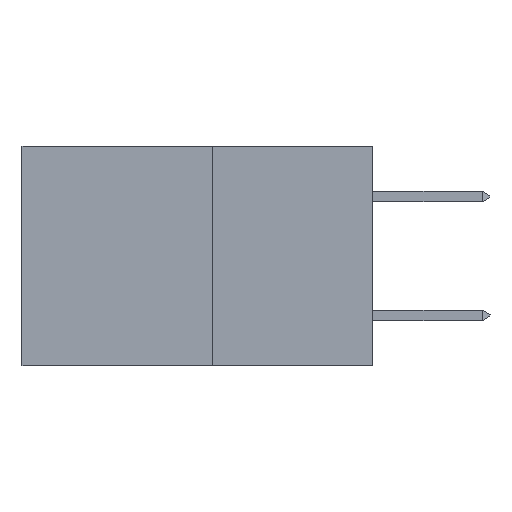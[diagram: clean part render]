
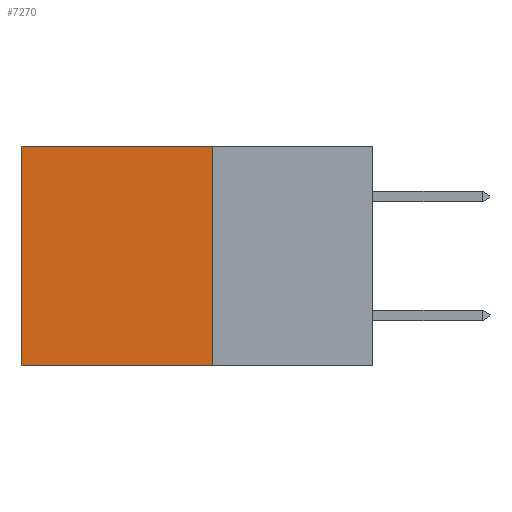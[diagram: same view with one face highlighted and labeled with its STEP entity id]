
A CAD part, left-side view. The second image highlights one B-rep face of the part: STEP entity #7270.
In plain terms, the highlighted planar face has unit normal (-1, 0, 0).
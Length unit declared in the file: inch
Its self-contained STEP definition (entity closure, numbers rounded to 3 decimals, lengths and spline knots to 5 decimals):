
#323 = CARTESIAN_POINT ( 'NONE',  ( 0.277, 0.59, 0. ) ) ;
#431 = EDGE_LOOP ( 'NONE', ( #13300, #8827, #19521, #10023 ) ) ;
#618 = EDGE_CURVE ( 'NONE', #21297, #9839, #15740, .T. ) ;
#1033 = DIRECTION ( 'NONE',  ( 0., 0., -1. ) ) ;
#2164 = CARTESIAN_POINT ( 'NONE',  ( 0.277, 0.59, -0.37 ) ) ;
#3839 = FACE_OUTER_BOUND ( 'NONE', #431, .T. ) ;
#4172 = VERTEX_POINT ( 'NONE', #14036 ) ;
#4552 = VECTOR ( 'NONE', #4832, 39.37008 ) ;
#4832 = DIRECTION ( 'NONE',  ( 0., 0., -1. ) ) ;
#5787 = VERTEX_POINT ( 'NONE', #10818 ) ;
#7270 = ADVANCED_FACE ( 'NONE', ( #3839 ), #23300, .F. ) ;
#8087 = DIRECTION ( 'NONE',  ( 0., 0., -1. ) ) ;
#8827 = ORIENTED_EDGE ( 'NONE', *, *, #24014, .F. ) ;
#9708 = LINE ( 'NONE', #20129, #4552 ) ;
#9839 = VERTEX_POINT ( 'NONE', #2164 ) ;
#10023 = ORIENTED_EDGE ( 'NONE', *, *, #21943, .T. ) ;
#10700 = VECTOR ( 'NONE', #8087, 39.37008 ) ;
#10818 = CARTESIAN_POINT ( 'NONE',  ( 0.277, 0.27, -0.37 ) ) ;
#13300 = ORIENTED_EDGE ( 'NONE', *, *, #618, .T. ) ;
#13712 = CARTESIAN_POINT ( 'NONE',  ( 0.277, 0.27, 0. ) ) ;
#14000 = LINE ( 'NONE', #23015, #24183 ) ;
#14036 = CARTESIAN_POINT ( 'NONE',  ( 0.277, 0.27, 0. ) ) ;
#15620 = DIRECTION ( 'NONE',  ( 0., 1., 0. ) ) ;
#15740 = LINE ( 'NONE', #17177, #10700 ) ;
#15846 = VECTOR ( 'NONE', #15620, 39.37008 ) ;
#17177 = CARTESIAN_POINT ( 'NONE',  ( 0.277, 0.59, -0.37 ) ) ;
#17493 = EDGE_CURVE ( 'NONE', #4172, #5787, #9708, .T. ) ;
#18399 = AXIS2_PLACEMENT_3D ( 'NONE', #19696, #23014, #1033 ) ;
#19521 = ORIENTED_EDGE ( 'NONE', *, *, #17493, .F. ) ;
#19696 = CARTESIAN_POINT ( 'NONE',  ( 0.277, 0.27, -0.37 ) ) ;
#20129 = CARTESIAN_POINT ( 'NONE',  ( 0.277, 0.27, -0.37 ) ) ;
#20903 = LINE ( 'NONE', #13712, #15846 ) ;
#21297 = VERTEX_POINT ( 'NONE', #323 ) ;
#21943 = EDGE_CURVE ( 'NONE', #4172, #21297, #20903, .T. ) ;
#23014 = DIRECTION ( 'NONE',  ( 1., 0., 0. ) ) ;
#23015 = CARTESIAN_POINT ( 'NONE',  ( 0.277, 0.27, -0.37 ) ) ;
#23300 = PLANE ( 'NONE',  #18399 ) ;
#24014 = EDGE_CURVE ( 'NONE', #5787, #9839, #14000, .T. ) ;
#24183 = VECTOR ( 'NONE', #24954, 39.37008 ) ;
#24954 = DIRECTION ( 'NONE',  ( 0., 1., 0. ) ) ;
